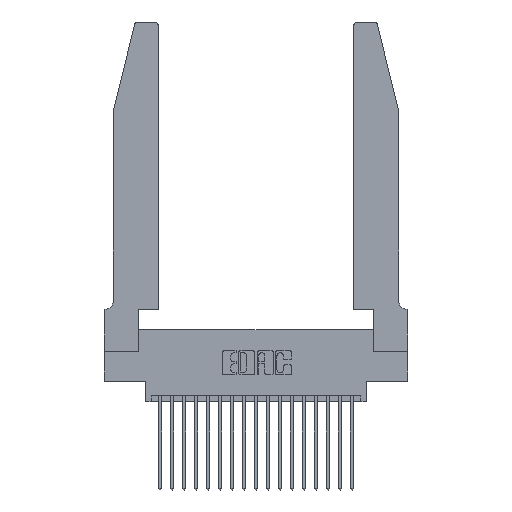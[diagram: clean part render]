
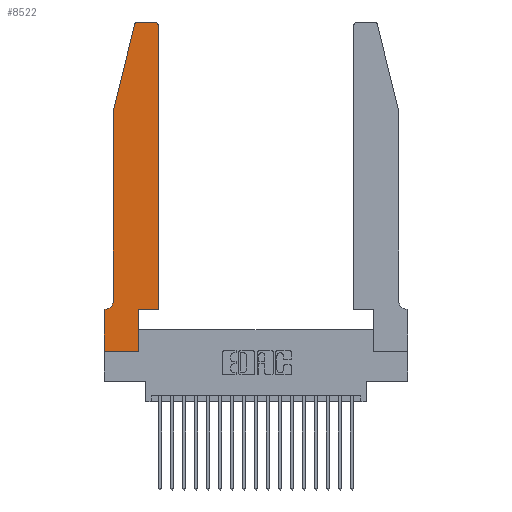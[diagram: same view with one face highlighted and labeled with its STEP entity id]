
A CAD part, top view. The second image highlights one B-rep face of the part: STEP entity #8522.
In plain terms, the highlighted planar face has unit normal (0, 0, 1).
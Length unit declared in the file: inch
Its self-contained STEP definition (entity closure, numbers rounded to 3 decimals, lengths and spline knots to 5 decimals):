
#167 = ORIENTED_EDGE ( 'NONE', *, *, #13273, .T. ) ;
#221 = EDGE_CURVE ( 'NONE', #4116, #3292, #17047, .T. ) ;
#401 = ORIENTED_EDGE ( 'NONE', *, *, #16036, .T. ) ;
#460 = CARTESIAN_POINT ( 'NONE',  ( 0., 0.35, 0.37 ) ) ;
#530 = ORIENTED_EDGE ( 'NONE', *, *, #6087, .T. ) ;
#579 = EDGE_CURVE ( 'NONE', #1772, #14857, #20042, .T. ) ;
#580 = CARTESIAN_POINT ( 'NONE',  ( 0.0055, 0.35, 0.37 ) ) ;
#746 = CARTESIAN_POINT ( 'NONE',  ( 0.2865, 0.35, 0.37 ) ) ;
#782 = ORIENTED_EDGE ( 'NONE', *, *, #5708, .T. ) ;
#1208 = VERTEX_POINT ( 'NONE', #11862 ) ;
#1437 = ORIENTED_EDGE ( 'NONE', *, *, #18671, .T. ) ;
#1701 = DIRECTION ( 'NONE',  ( -1., 0., 0. ) ) ;
#1772 = VERTEX_POINT ( 'NONE', #3721 ) ;
#1795 = ORIENTED_EDGE ( 'NONE', *, *, #17881, .T. ) ;
#1884 = CARTESIAN_POINT ( 'NONE',  ( 0.4505, 0.35, 0.37 ) ) ;
#2468 = ORIENTED_EDGE ( 'NONE', *, *, #8566, .T. ) ;
#2517 = ORIENTED_EDGE ( 'NONE', *, *, #579, .T. ) ;
#3030 = CARTESIAN_POINT ( 'NONE',  ( 0., 0., 0.37 ) ) ;
#3292 = VERTEX_POINT ( 'NONE', #8745 ) ;
#3352 = CIRCLE ( 'NONE', #10419, 0.03 ) ;
#3716 = ORIENTED_EDGE ( 'NONE', *, *, #7454, .T. ) ;
#3721 = CARTESIAN_POINT ( 'NONE',  ( 0.25487, 2.72718, 0.37 ) ) ;
#3886 = LINE ( 'NONE', #1884, #16645 ) ;
#3902 = VECTOR ( 'NONE', #10960, 39.37008 ) ;
#4116 = VERTEX_POINT ( 'NONE', #460 ) ;
#4505 = VERTEX_POINT ( 'NONE', #18190 ) ;
#4634 = ORIENTED_EDGE ( 'NONE', *, *, #221, .T. ) ;
#4668 = VERTEX_POINT ( 'NONE', #9069 ) ;
#4918 = DIRECTION ( 'NONE',  ( -1., 0., 0. ) ) ;
#4934 = CARTESIAN_POINT ( 'NONE',  ( 0.2865, 0.35, 0.37 ) ) ;
#5458 = VECTOR ( 'NONE', #4918, 39.37008 ) ;
#5543 = ORIENTED_EDGE ( 'NONE', *, *, #9276, .T. ) ;
#5621 = CARTESIAN_POINT ( 'NONE',  ( 0.4505, 0.35, 0.37 ) ) ;
#5708 = EDGE_CURVE ( 'NONE', #9684, #1772, #3352, .T. ) ;
#5750 = DIRECTION ( 'NONE',  ( 0., 0., 1. ) ) ;
#6087 = EDGE_CURVE ( 'NONE', #4505, #9684, #13825, .T. ) ;
#6474 = PLANE ( 'NONE',  #19144 ) ;
#6540 = CARTESIAN_POINT ( 'NONE',  ( 0.2865, 0., 0.37 ) ) ;
#6556 = DIRECTION ( 'NONE',  ( 0., 0., 1. ) ) ;
#6633 = DIRECTION ( 'NONE',  ( 0., 1., 0. ) ) ;
#6703 = VECTOR ( 'NONE', #1701, 39.37008 ) ;
#7163 = CARTESIAN_POINT ( 'NONE',  ( 0.0755, 2., 0.37 ) ) ;
#7173 = LINE ( 'NONE', #4934, #15487 ) ;
#7332 = DIRECTION ( 'NONE',  ( -0.239, -0.971, 0. ) ) ;
#7454 = EDGE_CURVE ( 'NONE', #1208, #4505, #10935, .T. ) ;
#7655 = CARTESIAN_POINT ( 'NONE',  ( 0.0055, 0.42, 0.37 ) ) ;
#8244 = CARTESIAN_POINT ( 'NONE',  ( 0.2605, 2.75, 0.37 ) ) ;
#8286 = VECTOR ( 'NONE', #17996, 39.37008 ) ;
#8380 = DIRECTION ( 'NONE',  ( 0., -1., 0. ) ) ;
#8522 = ADVANCED_FACE ( 'NONE', ( #16832 ), #6474, .T. ) ;
#8530 = ORIENTED_EDGE ( 'NONE', *, *, #18484, .T. ) ;
#8566 = EDGE_CURVE ( 'NONE', #14857, #4668, #19581, .T. ) ;
#8745 = CARTESIAN_POINT ( 'NONE',  ( 0., 0., 0.37 ) ) ;
#8752 = DIRECTION ( 'NONE',  ( 0., 1., 0. ) ) ;
#9069 = CARTESIAN_POINT ( 'NONE',  ( 0.0755, 0.42, 0.37 ) ) ;
#9137 = CARTESIAN_POINT ( 'NONE',  ( 0.4205, 2.72, 0.37 ) ) ;
#9272 = CARTESIAN_POINT ( 'NONE',  ( 0., 0., 0.37 ) ) ;
#9276 = EDGE_CURVE ( 'NONE', #14657, #4116, #10154, .T. ) ;
#9287 = EDGE_LOOP ( 'NONE', ( #530, #782, #2517, #2468, #1437, #5543, #4634, #167, #401, #1795, #8530, #3716 ) ) ;
#9342 = DIRECTION ( 'NONE',  ( -1., 0., 0. ) ) ;
#9684 = VERTEX_POINT ( 'NONE', #14511 ) ;
#10039 = CARTESIAN_POINT ( 'NONE',  ( 0.0755, 2., 0.37 ) ) ;
#10154 = LINE ( 'NONE', #13535, #6703 ) ;
#10419 = AXIS2_PLACEMENT_3D ( 'NONE', #15696, #5750, #17298 ) ;
#10824 = DIRECTION ( 'NONE',  ( 1., 0., 0. ) ) ;
#10935 = CIRCLE ( 'NONE', #14997, 0.03 ) ;
#10960 = DIRECTION ( 'NONE',  ( 1., 0., 0. ) ) ;
#11862 = CARTESIAN_POINT ( 'NONE',  ( 0.4505, 2.72, 0.37 ) ) ;
#12379 = AXIS2_PLACEMENT_3D ( 'NONE', #7655, #19110, #9342 ) ;
#12620 = CARTESIAN_POINT ( 'NONE',  ( 0.4505, 0.35, 0.37 ) ) ;
#13129 = CARTESIAN_POINT ( 'NONE',  ( 0.0755, 2., 0.37 ) ) ;
#13273 = EDGE_CURVE ( 'NONE', #3292, #14909, #13361, .T. ) ;
#13361 = LINE ( 'NONE', #9272, #3902 ) ;
#13535 = CARTESIAN_POINT ( 'NONE',  ( 0.0755, 0.35, 0.37 ) ) ;
#13825 = LINE ( 'NONE', #8244, #5458 ) ;
#14511 = CARTESIAN_POINT ( 'NONE',  ( 0.284, 2.75, 0.37 ) ) ;
#14657 = VERTEX_POINT ( 'NONE', #580 ) ;
#14857 = VERTEX_POINT ( 'NONE', #13129 ) ;
#14909 = VERTEX_POINT ( 'NONE', #6540 ) ;
#14997 = AXIS2_PLACEMENT_3D ( 'NONE', #9137, #20539, #10824 ) ;
#15319 = VECTOR ( 'NONE', #8380, 39.37008 ) ;
#15487 = VECTOR ( 'NONE', #6633, 39.37008 ) ;
#15696 = CARTESIAN_POINT ( 'NONE',  ( 0.284, 2.72, 0.37 ) ) ;
#15773 = VECTOR ( 'NONE', #7332, 39.37008 ) ;
#15906 = VECTOR ( 'NONE', #17187, 39.37008 ) ;
#16036 = EDGE_CURVE ( 'NONE', #14909, #18667, #7173, .T. ) ;
#16471 = CARTESIAN_POINT ( 'NONE',  ( 0., 0.35, 0.37 ) ) ;
#16645 = VECTOR ( 'NONE', #8752, 39.37008 ) ;
#16832 = FACE_OUTER_BOUND ( 'NONE', #9287, .T. ) ;
#17047 = LINE ( 'NONE', #3030, #8286 ) ;
#17187 = DIRECTION ( 'NONE',  ( 1., 0., 0. ) ) ;
#17298 = DIRECTION ( 'NONE',  ( 1., 0., 0. ) ) ;
#17359 = CIRCLE ( 'NONE', #12379, 0.07 ) ;
#17881 = EDGE_CURVE ( 'NONE', #18667, #18686, #19678, .T. ) ;
#17996 = DIRECTION ( 'NONE',  ( 0., -1., 0. ) ) ;
#18083 = DIRECTION ( 'NONE',  ( 1., 0., 0. ) ) ;
#18190 = CARTESIAN_POINT ( 'NONE',  ( 0.4205, 2.75, 0.37 ) ) ;
#18484 = EDGE_CURVE ( 'NONE', #18686, #1208, #3886, .T. ) ;
#18667 = VERTEX_POINT ( 'NONE', #746 ) ;
#18671 = EDGE_CURVE ( 'NONE', #4668, #14657, #17359, .T. ) ;
#18686 = VERTEX_POINT ( 'NONE', #12620 ) ;
#19110 = DIRECTION ( 'NONE',  ( 0., 0., -1. ) ) ;
#19144 = AXIS2_PLACEMENT_3D ( 'NONE', #16471, #6556, #18083 ) ;
#19581 = LINE ( 'NONE', #10039, #15319 ) ;
#19678 = LINE ( 'NONE', #5621, #15906 ) ;
#20042 = LINE ( 'NONE', #7163, #15773 ) ;
#20539 = DIRECTION ( 'NONE',  ( 0., 0., 1. ) ) ;
